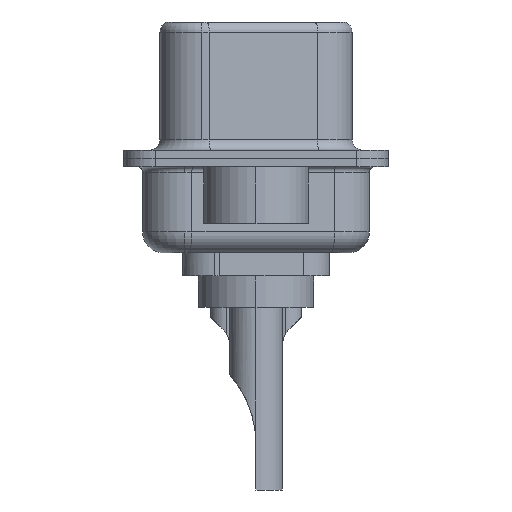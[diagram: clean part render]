
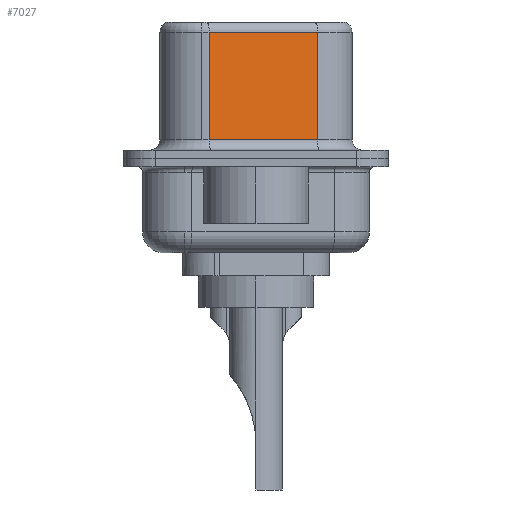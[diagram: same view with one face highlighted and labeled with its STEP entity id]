
A CAD part, left-side view. The second image highlights one B-rep face of the part: STEP entity #7027.
In plain terms, the highlighted planar face has unit normal (-0.985, -0.174, 0).
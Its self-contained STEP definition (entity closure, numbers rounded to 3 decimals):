
#197 = CARTESIAN_POINT ( 'NONE',  ( 3.675, 2.233, 6.02 ) ) ;
#1135 = DIRECTION ( 'NONE',  ( 0., 0., -1. ) ) ;
#1638 = VECTOR ( 'NONE', #1135, 1000. ) ;
#2829 = CARTESIAN_POINT ( 'NONE',  ( 3.675, 2.233, 0.9 ) ) ;
#3338 = CARTESIAN_POINT ( 'NONE',  ( 4.585, -2.927, 6.52 ) ) ;
#4718 = DIRECTION ( 'NONE',  ( 0., 0., -1. ) ) ;
#4805 = PLANE ( 'NONE',  #15743 ) ;
#4922 = VERTEX_POINT ( 'NONE', #197 ) ;
#5163 = DIRECTION ( 'NONE',  ( -0.174, 0.985, 0. ) ) ;
#5468 = VERTEX_POINT ( 'NONE', #10935 ) ;
#5630 = LINE ( 'NONE', #15422, #15429 ) ;
#6203 = DIRECTION ( 'NONE',  ( -0.174, 0.985, 0. ) ) ;
#6343 = ORIENTED_EDGE ( 'NONE', *, *, #9210, .T. ) ;
#6875 = ORIENTED_EDGE ( 'NONE', *, *, #10706, .T. ) ;
#7027 = ADVANCED_FACE ( 'NONE', ( #15295 ), #4805, .F. ) ;
#8890 = CARTESIAN_POINT ( 'NONE',  ( 4.585, -2.927, 6.52 ) ) ;
#9210 = EDGE_CURVE ( 'NONE', #12936, #5468, #5630, .T. ) ;
#10673 = CARTESIAN_POINT ( 'NONE',  ( 3.675, 2.233, 6.52 ) ) ;
#10706 = EDGE_CURVE ( 'NONE', #11655, #4922, #14597, .T. ) ;
#10900 = CARTESIAN_POINT ( 'NONE',  ( 4.585, -2.927, 6.02 ) ) ;
#10935 = CARTESIAN_POINT ( 'NONE',  ( 4.585, -2.927, 0.9 ) ) ;
#11123 = VECTOR ( 'NONE', #5163, 1000. ) ;
#11541 = DIRECTION ( 'NONE',  ( 0.174, -0.985, 0. ) ) ;
#11655 = VERTEX_POINT ( 'NONE', #10900 ) ;
#11936 = EDGE_CURVE ( 'NONE', #11655, #5468, #13312, .T. ) ;
#12425 = LINE ( 'NONE', #10673, #1638 ) ;
#12936 = VERTEX_POINT ( 'NONE', #2829 ) ;
#13312 = LINE ( 'NONE', #3338, #16851 ) ;
#13472 = EDGE_CURVE ( 'NONE', #4922, #12936, #12425, .T. ) ;
#14159 = DIRECTION ( 'NONE',  ( 0.985, 0.174, 0. ) ) ;
#14527 = CARTESIAN_POINT ( 'NONE',  ( 4.585, -2.927, 6.02 ) ) ;
#14597 = LINE ( 'NONE', #14527, #11123 ) ;
#15179 = ORIENTED_EDGE ( 'NONE', *, *, #13472, .T. ) ;
#15222 = ORIENTED_EDGE ( 'NONE', *, *, #11936, .F. ) ;
#15295 = FACE_OUTER_BOUND ( 'NONE', #16682, .T. ) ;
#15422 = CARTESIAN_POINT ( 'NONE',  ( 4.585, -2.927, 0.9 ) ) ;
#15429 = VECTOR ( 'NONE', #11541, 1000. ) ;
#15743 = AXIS2_PLACEMENT_3D ( 'NONE', #8890, #14159, #6203 ) ;
#16682 = EDGE_LOOP ( 'NONE', ( #15222, #6875, #15179, #6343 ) ) ;
#16851 = VECTOR ( 'NONE', #4718, 1000. ) ;
